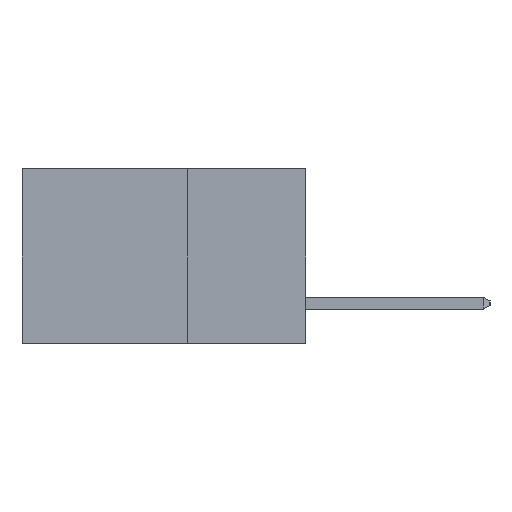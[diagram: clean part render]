
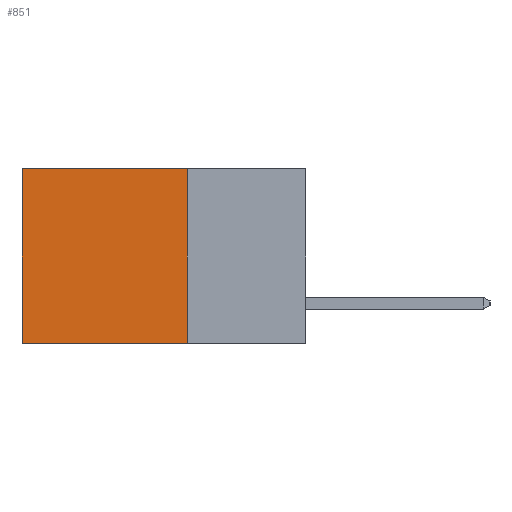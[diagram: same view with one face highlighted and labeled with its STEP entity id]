
A CAD part, left-side view. The second image highlights one B-rep face of the part: STEP entity #851.
In plain terms, the highlighted planar face has unit normal (-1, 0, 0).
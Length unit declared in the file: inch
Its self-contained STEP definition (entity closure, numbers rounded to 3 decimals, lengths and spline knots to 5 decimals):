
#851 = ADVANCED_FACE ( 'NONE', ( #17312 ), #10945, .F. ) ;
#1380 = CARTESIAN_POINT ( 'NONE',  ( 0.2615, 0.25, -0.37 ) ) ;
#1574 = DIRECTION ( 'NONE',  ( 0., 1., 0. ) ) ;
#1610 = DIRECTION ( 'NONE',  ( 0., 1., 0. ) ) ;
#2028 = VECTOR ( 'NONE', #5993, 39.37008 ) ;
#2766 = VERTEX_POINT ( 'NONE', #8953 ) ;
#3290 = CARTESIAN_POINT ( 'NONE',  ( 0.2615, 0.6, 0. ) ) ;
#4086 = EDGE_CURVE ( 'NONE', #2766, #8602, #14441, .T. ) ;
#5779 = CARTESIAN_POINT ( 'NONE',  ( 0.2615, 0.25, -0.37 ) ) ;
#5993 = DIRECTION ( 'NONE',  ( 0., 0., -1. ) ) ;
#7393 = VERTEX_POINT ( 'NONE', #8229 ) ;
#8229 = CARTESIAN_POINT ( 'NONE',  ( 0.2615, 0.6, -0.37 ) ) ;
#8414 = AXIS2_PLACEMENT_3D ( 'NONE', #10919, #10875, #10835 ) ;
#8602 = VERTEX_POINT ( 'NONE', #17679 ) ;
#8953 = CARTESIAN_POINT ( 'NONE',  ( 0.2615, 0.25, 0. ) ) ;
#10462 = EDGE_CURVE ( 'NONE', #8602, #7393, #13149, .T. ) ;
#10835 = DIRECTION ( 'NONE',  ( 0., 0., -1. ) ) ;
#10875 = DIRECTION ( 'NONE',  ( 1., 0., 0. ) ) ;
#10919 = CARTESIAN_POINT ( 'NONE',  ( 0.2615, 0.25, -0.37 ) ) ;
#10945 = PLANE ( 'NONE',  #8414 ) ;
#10974 = VECTOR ( 'NONE', #19140, 39.37008 ) ;
#11951 = EDGE_CURVE ( 'NONE', #16706, #7393, #15858, .T. ) ;
#12096 = ORIENTED_EDGE ( 'NONE', *, *, #11951, .T. ) ;
#13149 = LINE ( 'NONE', #1380, #16610 ) ;
#13314 = VECTOR ( 'NONE', #1610, 39.37008 ) ;
#13582 = CARTESIAN_POINT ( 'NONE',  ( 0.2615, 0.25, 0. ) ) ;
#13781 = LINE ( 'NONE', #13582, #13314 ) ;
#14441 = LINE ( 'NONE', #5779, #2028 ) ;
#15686 = ORIENTED_EDGE ( 'NONE', *, *, #4086, .F. ) ;
#15858 = LINE ( 'NONE', #17726, #10974 ) ;
#16346 = ORIENTED_EDGE ( 'NONE', *, *, #19075, .T. ) ;
#16610 = VECTOR ( 'NONE', #1574, 39.37008 ) ;
#16640 = EDGE_LOOP ( 'NONE', ( #12096, #19157, #15686, #16346 ) ) ;
#16706 = VERTEX_POINT ( 'NONE', #3290 ) ;
#17312 = FACE_OUTER_BOUND ( 'NONE', #16640, .T. ) ;
#17679 = CARTESIAN_POINT ( 'NONE',  ( 0.2615, 0.25, -0.37 ) ) ;
#17726 = CARTESIAN_POINT ( 'NONE',  ( 0.2615, 0.6, -0.37 ) ) ;
#19075 = EDGE_CURVE ( 'NONE', #2766, #16706, #13781, .T. ) ;
#19140 = DIRECTION ( 'NONE',  ( 0., 0., -1. ) ) ;
#19157 = ORIENTED_EDGE ( 'NONE', *, *, #10462, .F. ) ;
